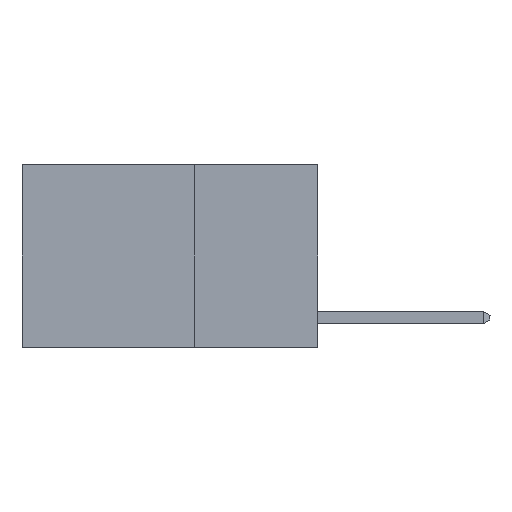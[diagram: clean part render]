
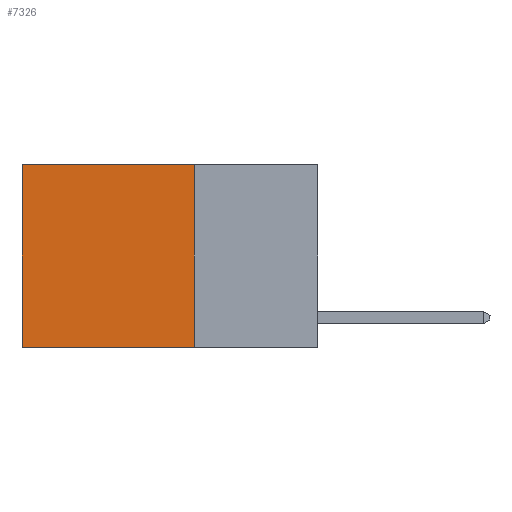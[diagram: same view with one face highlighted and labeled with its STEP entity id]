
A CAD part, left-side view. The second image highlights one B-rep face of the part: STEP entity #7326.
In plain terms, the highlighted planar face has unit normal (-1, 0, 0).
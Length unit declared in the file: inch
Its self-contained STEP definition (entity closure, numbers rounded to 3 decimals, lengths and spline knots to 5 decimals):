
#121 = VERTEX_POINT ( 'NONE', #705 ) ;
#705 = CARTESIAN_POINT ( 'NONE',  ( 0.2625, 0.25, -0.37 ) ) ;
#1176 = ORIENTED_EDGE ( 'NONE', *, *, #7660, .F. ) ;
#1464 = VERTEX_POINT ( 'NONE', #14130 ) ;
#1744 = DIRECTION ( 'NONE',  ( 1., 0., 0. ) ) ;
#1855 = CARTESIAN_POINT ( 'NONE',  ( 0.2625, 0.6, 0. ) ) ;
#2122 = CARTESIAN_POINT ( 'NONE',  ( 0.2625, 0.25, -0.37 ) ) ;
#2230 = ORIENTED_EDGE ( 'NONE', *, *, #3178, .T. ) ;
#2521 = VERTEX_POINT ( 'NONE', #11234 ) ;
#2743 = VECTOR ( 'NONE', #11739, 39.37008 ) ;
#2883 = LINE ( 'NONE', #11684, #2743 ) ;
#3178 = EDGE_CURVE ( 'NONE', #12036, #2521, #2883, .T. ) ;
#3249 = EDGE_LOOP ( 'NONE', ( #2230, #1176, #8367, #3845 ) ) ;
#3359 = LINE ( 'NONE', #11100, #13613 ) ;
#3475 = EDGE_CURVE ( 'NONE', #1464, #121, #3359, .T. ) ;
#3845 = ORIENTED_EDGE ( 'NONE', *, *, #6859, .T. ) ;
#3883 = DIRECTION ( 'NONE',  ( 0., 0., -1. ) ) ;
#4309 = FACE_OUTER_BOUND ( 'NONE', #3249, .T. ) ;
#4489 = LINE ( 'NONE', #2122, #10152 ) ;
#4622 = CARTESIAN_POINT ( 'NONE',  ( 0.2625, 0.25, 0. ) ) ;
#4672 = LINE ( 'NONE', #4622, #11936 ) ;
#5657 = DIRECTION ( 'NONE',  ( 0., 1., 0. ) ) ;
#6208 = PLANE ( 'NONE',  #8378 ) ;
#6859 = EDGE_CURVE ( 'NONE', #1464, #12036, #4672, .T. ) ;
#7326 = ADVANCED_FACE ( 'NONE', ( #4309 ), #6208, .F. ) ;
#7486 = CARTESIAN_POINT ( 'NONE',  ( 0.2625, 0.25, 0. ) ) ;
#7660 = EDGE_CURVE ( 'NONE', #121, #2521, #4489, .T. ) ;
#8367 = ORIENTED_EDGE ( 'NONE', *, *, #3475, .F. ) ;
#8378 = AXIS2_PLACEMENT_3D ( 'NONE', #7486, #1744, #3883 ) ;
#8911 = DIRECTION ( 'NONE',  ( 0., 0., -1. ) ) ;
#9045 = DIRECTION ( 'NONE',  ( 0., 1., 0. ) ) ;
#10152 = VECTOR ( 'NONE', #9045, 39.37008 ) ;
#11100 = CARTESIAN_POINT ( 'NONE',  ( 0.2625, 0.25, 0. ) ) ;
#11234 = CARTESIAN_POINT ( 'NONE',  ( 0.2625, 0.6, -0.37 ) ) ;
#11684 = CARTESIAN_POINT ( 'NONE',  ( 0.2625, 0.6, 0. ) ) ;
#11739 = DIRECTION ( 'NONE',  ( 0., 0., -1. ) ) ;
#11936 = VECTOR ( 'NONE', #5657, 39.37008 ) ;
#12036 = VERTEX_POINT ( 'NONE', #1855 ) ;
#13613 = VECTOR ( 'NONE', #8911, 39.37008 ) ;
#14130 = CARTESIAN_POINT ( 'NONE',  ( 0.2625, 0.25, 0. ) ) ;
